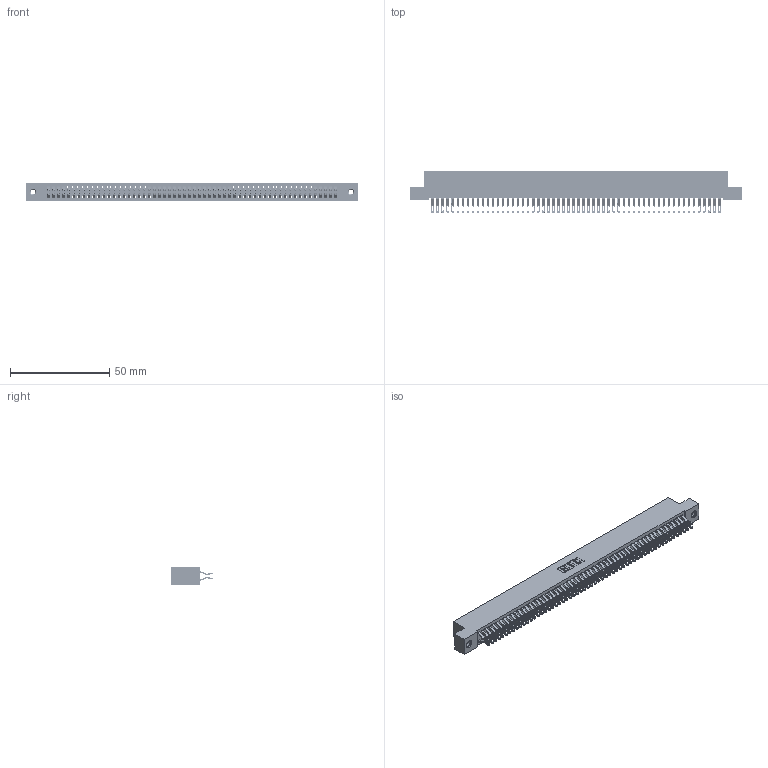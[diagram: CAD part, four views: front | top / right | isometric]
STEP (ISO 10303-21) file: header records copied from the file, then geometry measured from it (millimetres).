
FILE_DESCRIPTION (( 'STEP AP203' ), '1' );
FILE_NAME ('342-116-555-207.STEP', '2019-10-04T22:23:03', ( '' ), ( '' ), 'SwSTEP 2.0', 'SolidWorks 2016', '' );
FILE_SCHEMA (( 'CONFIG_CONTROL_DESIGN' ));
Length unit declared in the file: inch
Products named in the file (4): 342 Part_TI; 345-292-001_555 Tail; 345-250-001_345-250-005-103; 342-116-555-207
Assembly tree (119 placements, depth 2):
  342-116-555-207
    342 Part_TI
    345-292-001_555 Tail  x116
    345-250-001_345-250-005-103  x2
Bounding box: 167.64 x 21.47 x 9.4 mm (x, y, z)
Volume: 15447.8 mm3; surface area: 26687.6 mm2
Topology: 119 solids, 119 shells, 6898 faces, 21663 edges, 14434 vertices
Faces by surface type: plane 4042, cylinder 2840, cone 12, torus 4
Entity records: 36624 total; most frequent: CARTESIAN_POINT 6067, ORIENTED_EDGE 5966, DIRECTION 5157, EDGE_CURVE 2983, VECTOR 2815, LINE 2815, VERTEX_POINT 1984, AXIS2_PLACEMENT_3D 1171
